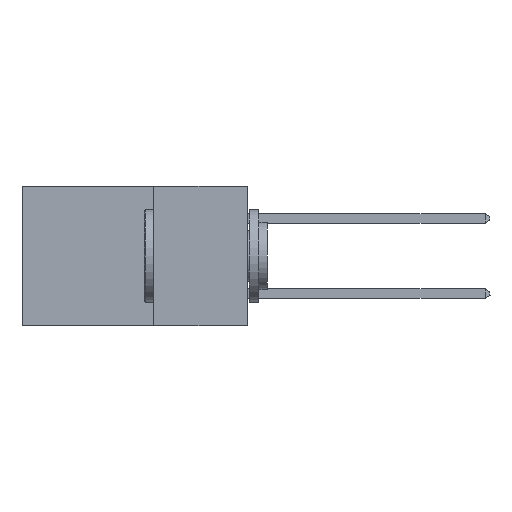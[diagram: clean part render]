
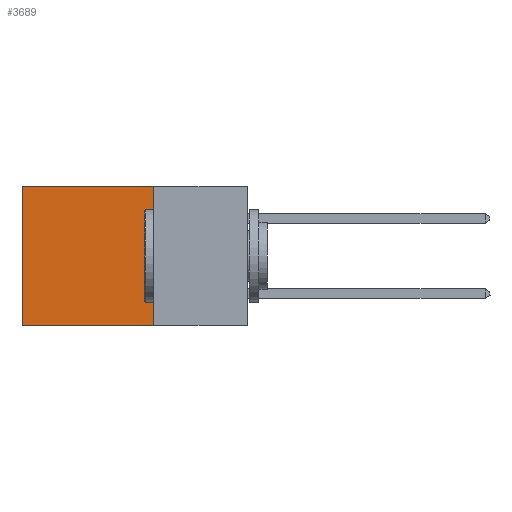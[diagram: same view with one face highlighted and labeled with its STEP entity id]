
A CAD part, left-side view. The second image highlights one B-rep face of the part: STEP entity #3689.
In plain terms, the highlighted planar face has unit normal (-1, 0, 0).
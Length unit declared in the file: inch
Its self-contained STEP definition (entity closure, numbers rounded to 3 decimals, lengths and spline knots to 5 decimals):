
#507 = DIRECTION ( 'NONE',  ( 0., 1., 0. ) ) ;
#585 = CARTESIAN_POINT ( 'NONE',  ( 0.298, 0.25, 0. ) ) ;
#1500 = VERTEX_POINT ( 'NONE', #10448 ) ;
#1780 = CARTESIAN_POINT ( 'NONE',  ( 0.298, 0.25, 0. ) ) ;
#2291 = VECTOR ( 'NONE', #9020, 39.37008 ) ;
#3689 = ADVANCED_FACE ( 'NONE', ( #12956 ), #18615, .F. ) ;
#4787 = DIRECTION ( 'NONE',  ( 0., 0., -1. ) ) ;
#4873 = ORIENTED_EDGE ( 'NONE', *, *, #12058, .F. ) ;
#4880 = LINE ( 'NONE', #585, #8788 ) ;
#5647 = EDGE_LOOP ( 'NONE', ( #10243, #17271, #4873, #7210 ) ) ;
#6595 = DIRECTION ( 'NONE',  ( 0., 1., 0. ) ) ;
#7076 = CARTESIAN_POINT ( 'NONE',  ( 0.298, 0.25, 0. ) ) ;
#7210 = ORIENTED_EDGE ( 'NONE', *, *, #12382, .T. ) ;
#8505 = CARTESIAN_POINT ( 'NONE',  ( 0.298, 0.25, -0.37 ) ) ;
#8522 = VERTEX_POINT ( 'NONE', #19869 ) ;
#8788 = VECTOR ( 'NONE', #507, 39.37008 ) ;
#8807 = VERTEX_POINT ( 'NONE', #9082 ) ;
#9020 = DIRECTION ( 'NONE',  ( 0., 0., -1. ) ) ;
#9082 = CARTESIAN_POINT ( 'NONE',  ( 0.298, 0.25, -0.37 ) ) ;
#9658 = VECTOR ( 'NONE', #4787, 39.37008 ) ;
#10001 = LINE ( 'NONE', #8505, #21215 ) ;
#10176 = DIRECTION ( 'NONE',  ( 0., 0., -1. ) ) ;
#10243 = ORIENTED_EDGE ( 'NONE', *, *, #16302, .T. ) ;
#10448 = CARTESIAN_POINT ( 'NONE',  ( 0.298, 0.6, 0. ) ) ;
#12058 = EDGE_CURVE ( 'NONE', #20400, #8807, #16875, .T. ) ;
#12382 = EDGE_CURVE ( 'NONE', #20400, #1500, #4880, .T. ) ;
#12956 = FACE_OUTER_BOUND ( 'NONE', #5647, .T. ) ;
#14865 = CARTESIAN_POINT ( 'NONE',  ( 0.298, 0.6, 0. ) ) ;
#15018 = EDGE_CURVE ( 'NONE', #8807, #8522, #10001, .T. ) ;
#15365 = DIRECTION ( 'NONE',  ( 1., 0., 0. ) ) ;
#15682 = CARTESIAN_POINT ( 'NONE',  ( 0.298, 0.25, 0. ) ) ;
#16302 = EDGE_CURVE ( 'NONE', #1500, #8522, #17768, .T. ) ;
#16875 = LINE ( 'NONE', #15682, #2291 ) ;
#17271 = ORIENTED_EDGE ( 'NONE', *, *, #15018, .F. ) ;
#17768 = LINE ( 'NONE', #14865, #9658 ) ;
#17863 = AXIS2_PLACEMENT_3D ( 'NONE', #1780, #15365, #10176 ) ;
#18615 = PLANE ( 'NONE',  #17863 ) ;
#19869 = CARTESIAN_POINT ( 'NONE',  ( 0.298, 0.6, -0.37 ) ) ;
#20400 = VERTEX_POINT ( 'NONE', #7076 ) ;
#21215 = VECTOR ( 'NONE', #6595, 39.37008 ) ;
